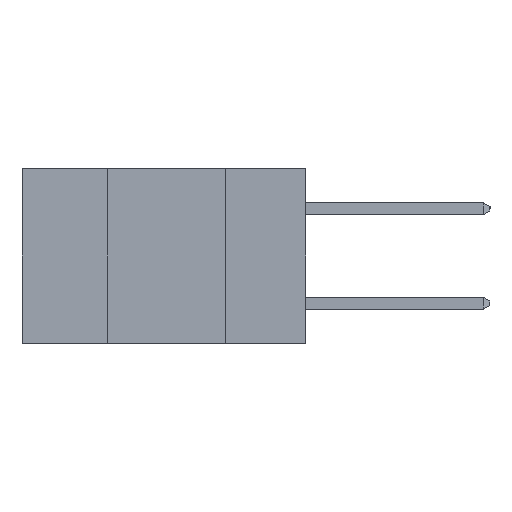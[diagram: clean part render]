
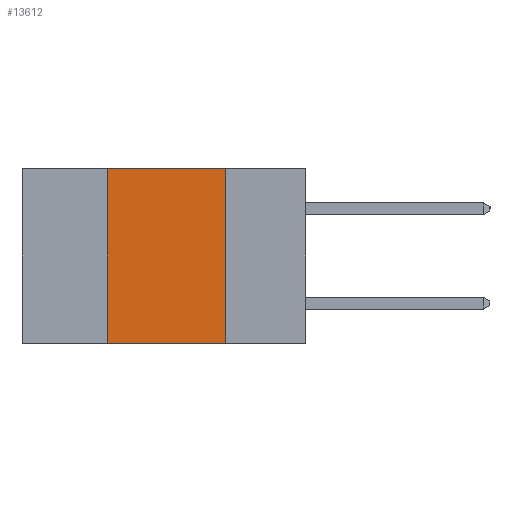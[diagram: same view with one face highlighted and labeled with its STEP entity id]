
A CAD part, left-side view. The second image highlights one B-rep face of the part: STEP entity #13612.
In plain terms, the highlighted planar face has unit normal (-1, 0, 0).
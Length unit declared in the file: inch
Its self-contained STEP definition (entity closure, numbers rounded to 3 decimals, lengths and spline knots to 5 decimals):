
#590 = LINE ( 'NONE', #9437, #3249 ) ;
#606 = EDGE_CURVE ( 'NONE', #697, #4709, #7453, .T. ) ;
#697 = VERTEX_POINT ( 'NONE', #3235 ) ;
#1172 = DIRECTION ( 'NONE',  ( 1., 0., 0. ) ) ;
#2121 = CARTESIAN_POINT ( 'NONE',  ( 0., 0.17, -0.37 ) ) ;
#2584 = LINE ( 'NONE', #13721, #7909 ) ;
#3235 = CARTESIAN_POINT ( 'NONE',  ( 0., 0.42, -0.37 ) ) ;
#3249 = VECTOR ( 'NONE', #8153, 39.37008 ) ;
#3523 = ORIENTED_EDGE ( 'NONE', *, *, #6936, .F. ) ;
#3860 = VERTEX_POINT ( 'NONE', #7398 ) ;
#4288 = EDGE_CURVE ( 'NONE', #697, #11619, #590, .T. ) ;
#4709 = VERTEX_POINT ( 'NONE', #6605 ) ;
#5026 = EDGE_LOOP ( 'NONE', ( #3523, #10651, #8050, #12246 ) ) ;
#6605 = CARTESIAN_POINT ( 'NONE',  ( 0., 0.17, -0.37 ) ) ;
#6628 = EDGE_CURVE ( 'NONE', #11619, #3860, #2584, .T. ) ;
#6936 = EDGE_CURVE ( 'NONE', #3860, #4709, #12355, .T. ) ;
#7398 = CARTESIAN_POINT ( 'NONE',  ( 0., 0.17, 0. ) ) ;
#7453 = LINE ( 'NONE', #14093, #12443 ) ;
#7609 = CARTESIAN_POINT ( 'NONE',  ( 0., 0.6, 0. ) ) ;
#7807 = DIRECTION ( 'NONE',  ( 0., 0., -1. ) ) ;
#7909 = VECTOR ( 'NONE', #8152, 39.37008 ) ;
#8050 = ORIENTED_EDGE ( 'NONE', *, *, #4288, .F. ) ;
#8152 = DIRECTION ( 'NONE',  ( 0., -1., 0. ) ) ;
#8153 = DIRECTION ( 'NONE',  ( 0., 0., 1. ) ) ;
#8639 = CARTESIAN_POINT ( 'NONE',  ( 0., 0.42, 0. ) ) ;
#8815 = FACE_OUTER_BOUND ( 'NONE', #5026, .T. ) ;
#9437 = CARTESIAN_POINT ( 'NONE',  ( 0., 0.42, -0.37 ) ) ;
#9802 = PLANE ( 'NONE',  #10723 ) ;
#10651 = ORIENTED_EDGE ( 'NONE', *, *, #6628, .F. ) ;
#10723 = AXIS2_PLACEMENT_3D ( 'NONE', #7609, #1172, #7807 ) ;
#11619 = VERTEX_POINT ( 'NONE', #8639 ) ;
#11906 = DIRECTION ( 'NONE',  ( 0., -1., 0. ) ) ;
#12246 = ORIENTED_EDGE ( 'NONE', *, *, #606, .T. ) ;
#12288 = DIRECTION ( 'NONE',  ( 0., 0., -1. ) ) ;
#12355 = LINE ( 'NONE', #2121, #13454 ) ;
#12443 = VECTOR ( 'NONE', #11906, 39.37008 ) ;
#13454 = VECTOR ( 'NONE', #12288, 39.37008 ) ;
#13612 = ADVANCED_FACE ( 'NONE', ( #8815 ), #9802, .F. ) ;
#13721 = CARTESIAN_POINT ( 'NONE',  ( 0., 0.6, 0. ) ) ;
#14093 = CARTESIAN_POINT ( 'NONE',  ( 0., 0.6, -0.37 ) ) ;
